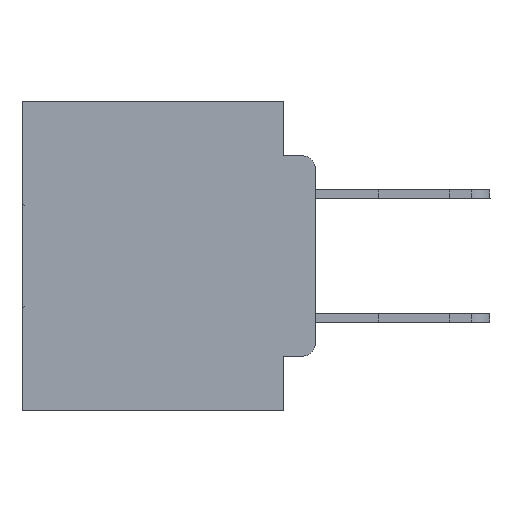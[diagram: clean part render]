
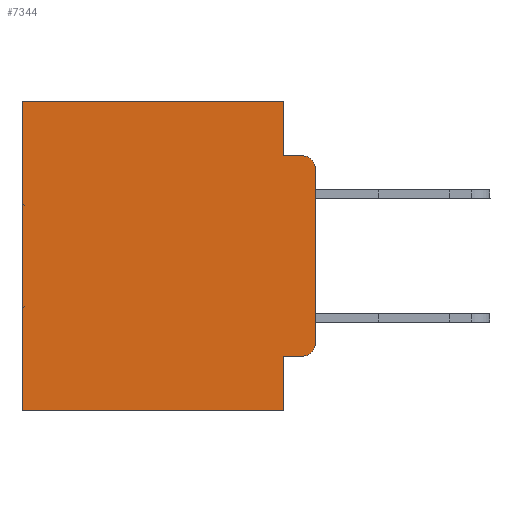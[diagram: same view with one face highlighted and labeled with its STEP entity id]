
A CAD part, left-side view. The second image highlights one B-rep face of the part: STEP entity #7344.
In plain terms, the highlighted planar face has unit normal (-1, 0, 0).
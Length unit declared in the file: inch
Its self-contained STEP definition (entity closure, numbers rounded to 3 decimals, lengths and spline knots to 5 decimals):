
#1156 = LINE ( 'NONE', #9274, #13676 ) ;
#1822 = DIRECTION ( 'NONE',  ( -1., 0., 0. ) ) ;
#2005 = CIRCLE ( 'NONE', #12057, 0.02 ) ;
#2379 = ORIENTED_EDGE ( 'NONE', *, *, #22314, .T. ) ;
#2746 = DIRECTION ( 'NONE',  ( 0., -1., 0. ) ) ;
#2839 = VERTEX_POINT ( 'NONE', #27358 ) ;
#3453 = VECTOR ( 'NONE', #16632, 39.37008 ) ;
#3474 = EDGE_CURVE ( 'NONE', #24696, #2839, #10081, .T. ) ;
#4694 = DIRECTION ( 'NONE',  ( 0., -1., 0. ) ) ;
#4787 = VECTOR ( 'NONE', #12727, 39.37008 ) ;
#5620 = VECTOR ( 'NONE', #11384, 39.37008 ) ;
#6396 = CARTESIAN_POINT ( 'NONE',  ( 0.298, 0.473, 0. ) ) ;
#7261 = LINE ( 'NONE', #29641, #20390 ) ;
#7344 = ADVANCED_FACE ( 'NONE', ( #24076 ), #19546, .F. ) ;
#8455 = LINE ( 'NONE', #13575, #14999 ) ;
#9274 = CARTESIAN_POINT ( 'NONE',  ( 0.298, 0., 0. ) ) ;
#9746 = CARTESIAN_POINT ( 'NONE',  ( 0.298, 0., 0. ) ) ;
#9896 = ORIENTED_EDGE ( 'NONE', *, *, #3474, .F. ) ;
#9920 = EDGE_CURVE ( 'NONE', #22756, #18718, #1156, .T. ) ;
#9996 = VERTEX_POINT ( 'NONE', #12073 ) ;
#10081 = LINE ( 'NONE', #18136, #3453 ) ;
#10610 = LINE ( 'NONE', #29946, #4787 ) ;
#10701 = EDGE_LOOP ( 'NONE', ( #9896, #14883, #19919, #14637, #28888, #2379, #17089, #15857, #15042, #22933 ) ) ;
#11384 = DIRECTION ( 'NONE',  ( 0., 0., -1. ) ) ;
#11495 = VERTEX_POINT ( 'NONE', #12623 ) ;
#12057 = AXIS2_PLACEMENT_3D ( 'NONE', #16723, #1822, #19222 ) ;
#12073 = CARTESIAN_POINT ( 'NONE',  ( 0.298, 0.02, -0.4115 ) ) ;
#12096 = VECTOR ( 'NONE', #2746, 39.37008 ) ;
#12219 = DIRECTION ( 'NONE',  ( 1., 0., 0. ) ) ;
#12385 = CARTESIAN_POINT ( 'NONE',  ( 0.298, 0.051, -0.5 ) ) ;
#12623 = CARTESIAN_POINT ( 'NONE',  ( 0.298, 0.02, -0.0885 ) ) ;
#12727 = DIRECTION ( 'NONE',  ( 0., 0., -1. ) ) ;
#13575 = CARTESIAN_POINT ( 'NONE',  ( 0.298, 0.051, 0. ) ) ;
#13676 = VECTOR ( 'NONE', #31328, 39.37008 ) ;
#13756 = LINE ( 'NONE', #6396, #5620 ) ;
#14278 = CARTESIAN_POINT ( 'NONE',  ( 0.298, 0.02, -0.1085 ) ) ;
#14637 = ORIENTED_EDGE ( 'NONE', *, *, #23972, .F. ) ;
#14883 = ORIENTED_EDGE ( 'NONE', *, *, #30455, .T. ) ;
#14988 = DIRECTION ( 'NONE',  ( 0., 1., 0. ) ) ;
#14999 = VECTOR ( 'NONE', #16029, 39.37008 ) ;
#15042 = ORIENTED_EDGE ( 'NONE', *, *, #19028, .T. ) ;
#15079 = LINE ( 'NONE', #21961, #27368 ) ;
#15513 = CARTESIAN_POINT ( 'NONE',  ( 0.298, 0.051, 0. ) ) ;
#15569 = EDGE_CURVE ( 'NONE', #18562, #29381, #7261, .T. ) ;
#15857 = ORIENTED_EDGE ( 'NONE', *, *, #20694, .F. ) ;
#16029 = DIRECTION ( 'NONE',  ( 0., 0., -1. ) ) ;
#16632 = DIRECTION ( 'NONE',  ( 0., 0., -1. ) ) ;
#16723 = CARTESIAN_POINT ( 'NONE',  ( 0.298, 0.02, -0.3915 ) ) ;
#16742 = DIRECTION ( 'NONE',  ( 0., 0., -1. ) ) ;
#16902 = CIRCLE ( 'NONE', #26317, 0.02 ) ;
#17089 = ORIENTED_EDGE ( 'NONE', *, *, #15569, .F. ) ;
#17346 = EDGE_CURVE ( 'NONE', #9996, #2839, #2005, .T. ) ;
#17534 = CARTESIAN_POINT ( 'NONE',  ( 0.298, 0.051, -0.0885 ) ) ;
#17863 = LINE ( 'NONE', #20115, #12096 ) ;
#18136 = CARTESIAN_POINT ( 'NONE',  ( 0.298, 0., 0. ) ) ;
#18562 = VERTEX_POINT ( 'NONE', #12385 ) ;
#18718 = VERTEX_POINT ( 'NONE', #30472 ) ;
#19028 = EDGE_CURVE ( 'NONE', #24702, #9996, #15079, .T. ) ;
#19222 = DIRECTION ( 'NONE',  ( 0., 0., -1. ) ) ;
#19546 = PLANE ( 'NONE',  #21907 ) ;
#19919 = ORIENTED_EDGE ( 'NONE', *, *, #27217, .F. ) ;
#20115 = CARTESIAN_POINT ( 'NONE',  ( 0.298, 0.051, -0.0885 ) ) ;
#20390 = VECTOR ( 'NONE', #14988, 39.37008 ) ;
#20694 = EDGE_CURVE ( 'NONE', #24702, #18562, #8455, .T. ) ;
#21907 = AXIS2_PLACEMENT_3D ( 'NONE', #9746, #12219, #29338 ) ;
#21961 = CARTESIAN_POINT ( 'NONE',  ( 0.298, 0.051, -0.4115 ) ) ;
#22314 = EDGE_CURVE ( 'NONE', #18718, #29381, #13756, .T. ) ;
#22756 = VERTEX_POINT ( 'NONE', #15513 ) ;
#22933 = ORIENTED_EDGE ( 'NONE', *, *, #17346, .T. ) ;
#23159 = CARTESIAN_POINT ( 'NONE',  ( 0.298, 0.051, -0.4115 ) ) ;
#23447 = CARTESIAN_POINT ( 'NONE',  ( 0.298, 0.473, -0.5 ) ) ;
#23972 = EDGE_CURVE ( 'NONE', #22756, #28529, #10610, .T. ) ;
#24076 = FACE_OUTER_BOUND ( 'NONE', #10701, .T. ) ;
#24696 = VERTEX_POINT ( 'NONE', #30334 ) ;
#24702 = VERTEX_POINT ( 'NONE', #23159 ) ;
#26317 = AXIS2_PLACEMENT_3D ( 'NONE', #14278, #31381, #16742 ) ;
#27217 = EDGE_CURVE ( 'NONE', #28529, #11495, #17863, .T. ) ;
#27358 = CARTESIAN_POINT ( 'NONE',  ( 0.298, 0., -0.3915 ) ) ;
#27368 = VECTOR ( 'NONE', #4694, 39.37008 ) ;
#28529 = VERTEX_POINT ( 'NONE', #17534 ) ;
#28888 = ORIENTED_EDGE ( 'NONE', *, *, #9920, .T. ) ;
#29338 = DIRECTION ( 'NONE',  ( 0., 0., -1. ) ) ;
#29381 = VERTEX_POINT ( 'NONE', #23447 ) ;
#29641 = CARTESIAN_POINT ( 'NONE',  ( 0.298, 0., -0.5 ) ) ;
#29946 = CARTESIAN_POINT ( 'NONE',  ( 0.298, 0.051, 0. ) ) ;
#30334 = CARTESIAN_POINT ( 'NONE',  ( 0.298, 0., -0.1085 ) ) ;
#30455 = EDGE_CURVE ( 'NONE', #24696, #11495, #16902, .T. ) ;
#30472 = CARTESIAN_POINT ( 'NONE',  ( 0.298, 0.473, 0. ) ) ;
#31328 = DIRECTION ( 'NONE',  ( 0., 1., 0. ) ) ;
#31381 = DIRECTION ( 'NONE',  ( -1., 0., 0. ) ) ;
